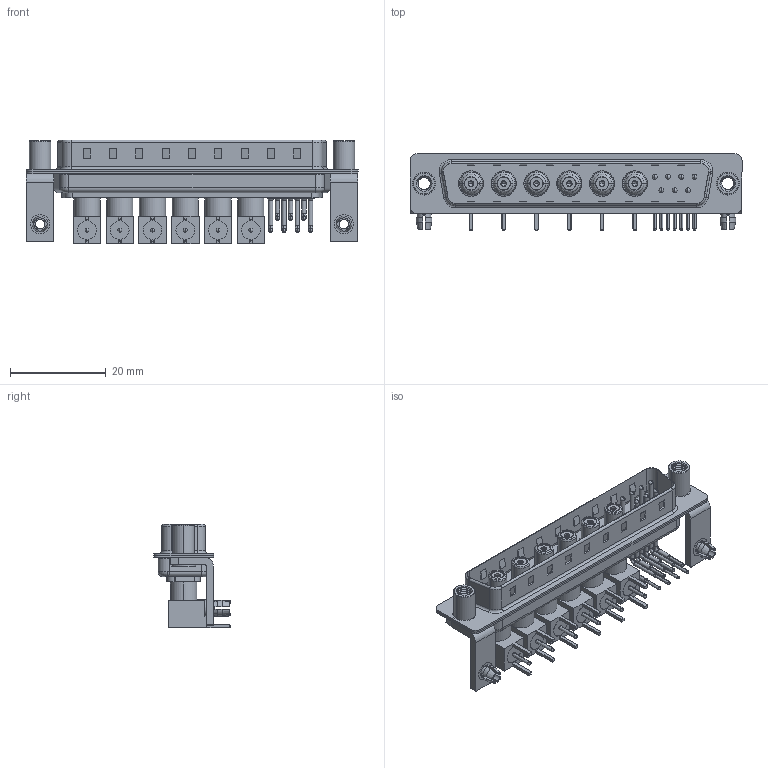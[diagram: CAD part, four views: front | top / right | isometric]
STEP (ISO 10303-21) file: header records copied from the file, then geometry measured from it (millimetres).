
FILE_DESCRIPTION (( 'STEP AP203' ), '1' );
FILE_NAME ('629-13W6240-7TD.STEP', '2022-05-14T14:53:06', ( '' ), ( '' ), 'SwSTEP 2.0', 'SolidWorks 2020', '' );
FILE_SCHEMA (( 'CONFIG_CONTROL_DESIGN' ));
Length unit declared in the file: millimetre
Products named in the file (22): Locking Collar; Co-Ax Jack_RA PC Tail; 629Combo Contact Row 2; Co-Ax Jack Assy_RA; RA Back Shell; 629Combo Threaded Standoff_D; Insulator Socket; Socket_RA; 629Combo Contact Row 1; 629Combo Stabilizer Bracket; 629Combo Shell Rear_37 Contacts; 629Combo Shell Front_37 Contacts; 629-13W6240-7TD; 629Combo Housing_13W6; Insulator Socket 2; Insulator RA Pin; 629Combo Board Lock
Assembly tree (64 placements, depth 3):
  629-13W6240-7TD
    629Combo Housing_13W6
    629Combo Shell Rear_37 Contacts
    629Combo Shell Front_37 Contacts
    629Combo Stabilizer Bracket  x2
    629Combo Board Lock  x2
    629Combo Threaded Standoff_D  x2
    Co-Ax Jack Assy_RA
      Co-Ax Jack_RA PC Tail
      Insulator Socket
      Insulator Socket 2
      Locking Collar
      Socket_RA
      RA Back Shell
      Insulator RA Pin
    Co-Ax Jack Assy_RA
      Co-Ax Jack_RA PC Tail
      Insulator Socket
      Insulator Socket 2
      Locking Collar
      Socket_RA
      RA Back Shell
      Insulator RA Pin
    Co-Ax Jack Assy_RA
      Co-Ax Jack_RA PC Tail
      Insulator Socket
      Insulator Socket 2
      Locking Collar
      Socket_RA
      RA Back Shell
      Insulator RA Pin
    Co-Ax Jack Assy_RA
      Co-Ax Jack_RA PC Tail
      Insulator Socket
      Insulator Socket 2
      Locking Collar
      Socket_RA
      RA Back Shell
      Insulator RA Pin
    Co-Ax Jack Assy_RA
      Co-Ax Jack_RA PC Tail
      Insulator Socket
      Insulator Socket 2
      Locking Collar
      Socket_RA
      RA Back Shell
      Insulator RA Pin
    Co-Ax Jack Assy_RA
      Co-Ax Jack_RA PC Tail
      Insulator Socket
      Insulator Socket 2
      Locking Collar
      Socket_RA
      RA Back Shell
      Insulator RA Pin
    629Combo Contact Row 1  x4
    629Combo Contact Row 2  x3
Bounding box: 69.4 x 16 x 21.71 mm (x, y, z)
Volume: 5957.1 mm3; surface area: 16085.7 mm2
Topology: 58 solids, 58 shells, 2284 faces, 5819 edges, 3704 vertices
Faces by surface type: plane 1063, cylinder 899, cone 170, torus 86, bspline 54, sphere 12
Entity records: 33991 total; most frequent: CARTESIAN_POINT 7629, DIRECTION 4964, ORIENTED_EDGE 4660, EDGE_CURVE 2330, AXIS2_PLACEMENT_3D 1782, VERTEX_POINT 1500, VECTOR 1400, LINE 1400
